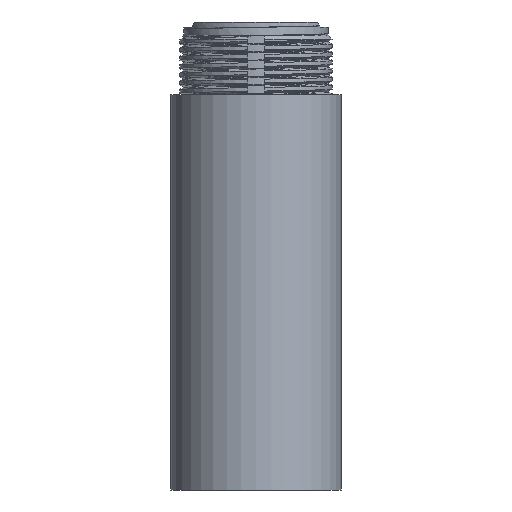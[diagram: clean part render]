
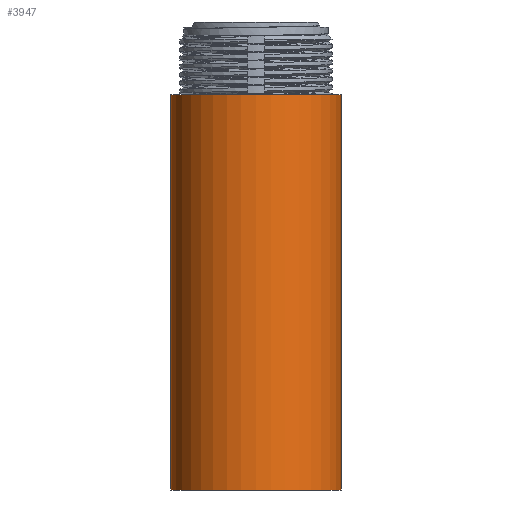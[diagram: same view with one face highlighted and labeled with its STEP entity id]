
A CAD part, front view. The second image highlights one B-rep face of the part: STEP entity #3947.
In plain terms, the highlighted cylindrical face has radius 16.383 mm (diameter 32.766 mm), a partial arc.
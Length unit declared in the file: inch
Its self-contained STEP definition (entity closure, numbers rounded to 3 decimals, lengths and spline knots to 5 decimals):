
#193 = AXIS2_PLACEMENT_3D ( 'NONE', #5955, #5936, #5934 ) ;
#524 = EDGE_CURVE ( 'NONE', #7721, #7596, #2840, .T. ) ;
#583 = EDGE_CURVE ( 'NONE', #7596, #6489, #2794, .T. ) ;
#669 = VECTOR ( 'NONE', #7956, 39.37008 ) ;
#814 = EDGE_CURVE ( 'NONE', #6489, #6664, #2640, .T. ) ;
#888 = CARTESIAN_POINT ( 'NONE',  ( -0.645, 0., 0.485 ) ) ;
#1011 = CYLINDRICAL_SURFACE ( 'NONE', #193, 0.645 ) ;
#1056 = EDGE_CURVE ( 'NONE', #7721, #6664, #2275, .T. ) ;
#1069 = FACE_OUTER_BOUND ( 'NONE', #5167, .T. ) ;
#1285 = CARTESIAN_POINT ( 'NONE',  ( 0., 0., -1.125 ) ) ;
#1296 = DIRECTION ( 'NONE',  ( 1., 0., 0. ) ) ;
#1300 = DIRECTION ( 'NONE',  ( 0., 0., -1. ) ) ;
#2266 = VECTOR ( 'NONE', #2935, 39.37008 ) ;
#2275 = LINE ( 'NONE', #2990, #2266 ) ;
#2640 = CIRCLE ( 'NONE', #4338, 0.645 ) ;
#2794 = LINE ( 'NONE', #888, #669 ) ;
#2840 = CIRCLE ( 'NONE', #4787, 0.645 ) ;
#2935 = DIRECTION ( 'NONE',  ( 0., 0., -1. ) ) ;
#2990 = CARTESIAN_POINT ( 'NONE',  ( 0.645, 0., 0.485 ) ) ;
#3734 = ORIENTED_EDGE ( 'NONE', *, *, #524, .T. ) ;
#3786 = ORIENTED_EDGE ( 'NONE', *, *, #583, .T. ) ;
#3794 = ORIENTED_EDGE ( 'NONE', *, *, #1056, .F. ) ;
#3947 = ADVANCED_FACE ( 'NONE', ( #1069 ), #1011, .T. ) ;
#4060 = CARTESIAN_POINT ( 'NONE',  ( 0.645, 0., -4.11042 ) ) ;
#4338 = AXIS2_PLACEMENT_3D ( 'NONE', #5436, #5412, #5376 ) ;
#4482 = ORIENTED_EDGE ( 'NONE', *, *, #814, .T. ) ;
#4787 = AXIS2_PLACEMENT_3D ( 'NONE', #1285, #1300, #1296 ) ;
#5167 = EDGE_LOOP ( 'NONE', ( #3734, #3786, #4482, #3794 ) ) ;
#5269 = CARTESIAN_POINT ( 'NONE',  ( 0.645, 0., -1.125 ) ) ;
#5376 = DIRECTION ( 'NONE',  ( -1., 0., 0. ) ) ;
#5412 = DIRECTION ( 'NONE',  ( 0., 0., 1. ) ) ;
#5436 = CARTESIAN_POINT ( 'NONE',  ( 0., 0., -4.11042 ) ) ;
#5934 = DIRECTION ( 'NONE',  ( 1., 0., 0. ) ) ;
#5936 = DIRECTION ( 'NONE',  ( 0., 0., -1. ) ) ;
#5955 = CARTESIAN_POINT ( 'NONE',  ( 0., 0., 0.485 ) ) ;
#6489 = VERTEX_POINT ( 'NONE', #7279 ) ;
#6501 = CARTESIAN_POINT ( 'NONE',  ( -0.645, 0., -1.125 ) ) ;
#6664 = VERTEX_POINT ( 'NONE', #4060 ) ;
#7279 = CARTESIAN_POINT ( 'NONE',  ( -0.645, 0., -4.11042 ) ) ;
#7596 = VERTEX_POINT ( 'NONE', #6501 ) ;
#7721 = VERTEX_POINT ( 'NONE', #5269 ) ;
#7956 = DIRECTION ( 'NONE',  ( 0., 0., -1. ) ) ;
